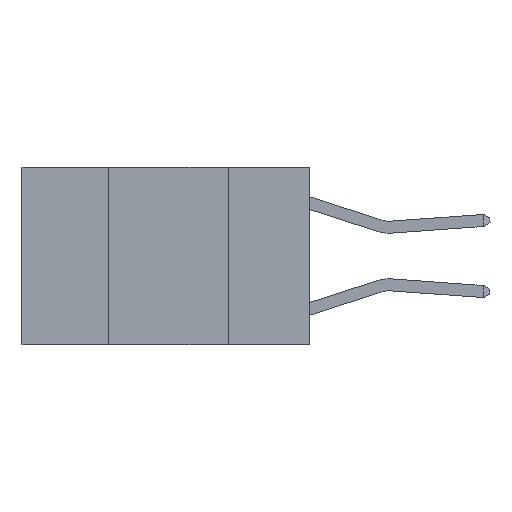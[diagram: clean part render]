
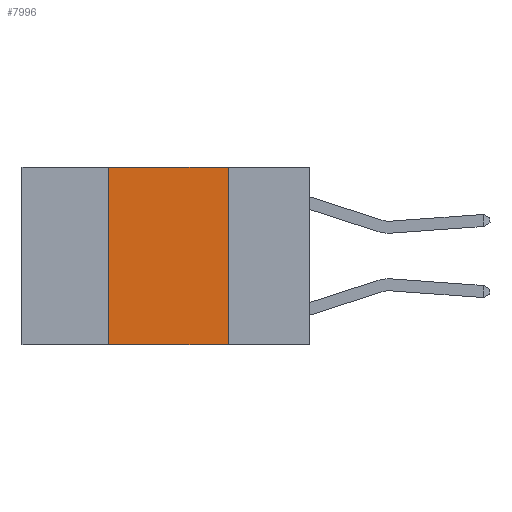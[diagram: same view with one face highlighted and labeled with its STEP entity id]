
A CAD part, left-side view. The second image highlights one B-rep face of the part: STEP entity #7996.
In plain terms, the highlighted planar face has unit normal (-1, 0, 0).
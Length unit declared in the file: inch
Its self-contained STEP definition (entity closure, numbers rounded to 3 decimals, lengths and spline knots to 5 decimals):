
#40 = DIRECTION ( 'NONE',  ( 0., 0., -1. ) ) ;
#78 = DIRECTION ( 'NONE',  ( 0., 0., 1. ) ) ;
#417 = EDGE_CURVE ( 'NONE', #3915, #5344, #5403, .T. ) ;
#603 = CARTESIAN_POINT ( 'NONE',  ( 0., 0.17, 0. ) ) ;
#849 = CARTESIAN_POINT ( 'NONE',  ( 0., 0.42, -0.37 ) ) ;
#1037 = LINE ( 'NONE', #8794, #4436 ) ;
#1428 = PLANE ( 'NONE',  #3600 ) ;
#1443 = FACE_OUTER_BOUND ( 'NONE', #6771, .T. ) ;
#1523 = LINE ( 'NONE', #2845, #8415 ) ;
#1626 = VECTOR ( 'NONE', #40, 39.37008 ) ;
#2088 = DIRECTION ( 'NONE',  ( 0., -1., 0. ) ) ;
#2404 = ORIENTED_EDGE ( 'NONE', *, *, #417, .F. ) ;
#2536 = ORIENTED_EDGE ( 'NONE', *, *, #3898, .F. ) ;
#2694 = DIRECTION ( 'NONE',  ( 0., -1., 0. ) ) ;
#2785 = ORIENTED_EDGE ( 'NONE', *, *, #6358, .F. ) ;
#2845 = CARTESIAN_POINT ( 'NONE',  ( 0., 0.6, 0. ) ) ;
#3034 = ORIENTED_EDGE ( 'NONE', *, *, #4524, .T. ) ;
#3600 = AXIS2_PLACEMENT_3D ( 'NONE', #5670, #8331, #4318 ) ;
#3898 = EDGE_CURVE ( 'NONE', #7461, #3915, #1523, .T. ) ;
#3915 = VERTEX_POINT ( 'NONE', #603 ) ;
#4318 = DIRECTION ( 'NONE',  ( 0., 0., -1. ) ) ;
#4436 = VECTOR ( 'NONE', #2694, 39.37008 ) ;
#4524 = EDGE_CURVE ( 'NONE', #8218, #5344, #1037, .T. ) ;
#4987 = CARTESIAN_POINT ( 'NONE',  ( 0., 0.17, -0.37 ) ) ;
#5344 = VERTEX_POINT ( 'NONE', #4987 ) ;
#5403 = LINE ( 'NONE', #6597, #1626 ) ;
#5670 = CARTESIAN_POINT ( 'NONE',  ( 0., 0.6, 0. ) ) ;
#5845 = CARTESIAN_POINT ( 'NONE',  ( 0., 0.42, 0. ) ) ;
#5889 = CARTESIAN_POINT ( 'NONE',  ( 0., 0.42, 0. ) ) ;
#5903 = LINE ( 'NONE', #5845, #7458 ) ;
#6358 = EDGE_CURVE ( 'NONE', #8218, #7461, #5903, .T. ) ;
#6597 = CARTESIAN_POINT ( 'NONE',  ( 0., 0.17, 0. ) ) ;
#6771 = EDGE_LOOP ( 'NONE', ( #2404, #2536, #2785, #3034 ) ) ;
#7458 = VECTOR ( 'NONE', #78, 39.37008 ) ;
#7461 = VERTEX_POINT ( 'NONE', #5889 ) ;
#7996 = ADVANCED_FACE ( 'NONE', ( #1443 ), #1428, .F. ) ;
#8218 = VERTEX_POINT ( 'NONE', #849 ) ;
#8331 = DIRECTION ( 'NONE',  ( 1., 0., 0. ) ) ;
#8415 = VECTOR ( 'NONE', #2088, 39.37008 ) ;
#8794 = CARTESIAN_POINT ( 'NONE',  ( 0., 0.6, -0.37 ) ) ;
